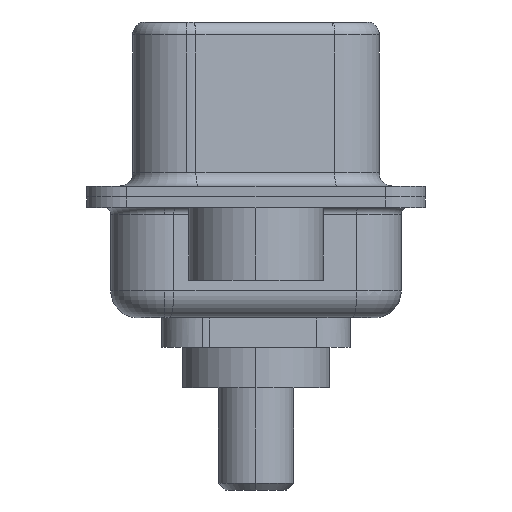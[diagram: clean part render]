
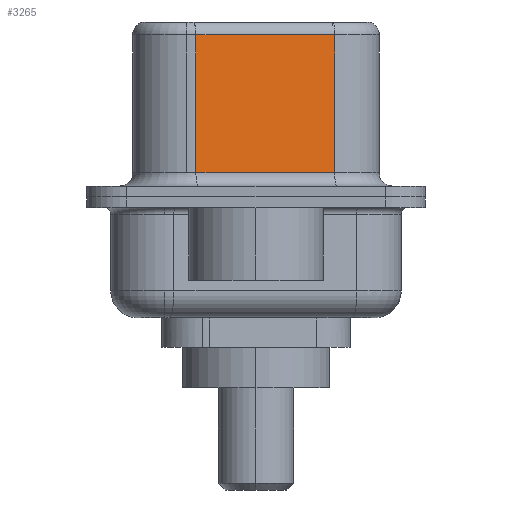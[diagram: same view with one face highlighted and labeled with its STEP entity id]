
A CAD part, left-side view. The second image highlights one B-rep face of the part: STEP entity #3265.
In plain terms, the highlighted planar face has unit normal (-0.985, -0.174, 0).
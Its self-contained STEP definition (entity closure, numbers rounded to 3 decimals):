
#342 = LINE ( 'NONE', #15076, #3213 ) ;
#769 = ORIENTED_EDGE ( 'NONE', *, *, #2416, .T. ) ;
#1430 = VECTOR ( 'NONE', #7669, 1000. ) ;
#1435 = EDGE_CURVE ( 'NONE', #5504, #11546, #342, .T. ) ;
#1739 = ORIENTED_EDGE ( 'NONE', *, *, #15233, .F. ) ;
#2416 = EDGE_CURVE ( 'NONE', #11546, #12562, #7179, .T. ) ;
#3213 = VECTOR ( 'NONE', #15706, 1000. ) ;
#3265 = ADVANCED_FACE ( 'NONE', ( #5222 ), #5969, .F. ) ;
#4072 = CARTESIAN_POINT ( 'NONE',  ( 4.58, -2.927, 6.52 ) ) ;
#5222 = FACE_OUTER_BOUND ( 'NONE', #7385, .T. ) ;
#5429 = DIRECTION ( 'NONE',  ( 0.174, -0.985, 0. ) ) ;
#5481 = LINE ( 'NONE', #11770, #8180 ) ;
#5504 = VERTEX_POINT ( 'NONE', #7075 ) ;
#5969 = PLANE ( 'NONE',  #13136 ) ;
#5988 = CARTESIAN_POINT ( 'NONE',  ( 3.67, 2.233, 6.02 ) ) ;
#6196 = CARTESIAN_POINT ( 'NONE',  ( 4.58, -2.927, 0.9 ) ) ;
#7075 = CARTESIAN_POINT ( 'NONE',  ( 4.58, -2.927, 6.02 ) ) ;
#7142 = CARTESIAN_POINT ( 'NONE',  ( 4.58, -2.927, 6.52 ) ) ;
#7179 = LINE ( 'NONE', #14147, #14959 ) ;
#7385 = EDGE_LOOP ( 'NONE', ( #1739, #12384, #769, #7457 ) ) ;
#7457 = ORIENTED_EDGE ( 'NONE', *, *, #14735, .T. ) ;
#7669 = DIRECTION ( 'NONE',  ( 0., 0., -1. ) ) ;
#8180 = VECTOR ( 'NONE', #5429, 1000. ) ;
#9249 = VERTEX_POINT ( 'NONE', #6196 ) ;
#9379 = LINE ( 'NONE', #4072, #1430 ) ;
#10450 = DIRECTION ( 'NONE',  ( 0., 0., -1. ) ) ;
#10930 = DIRECTION ( 'NONE',  ( 0.985, 0.174, 0. ) ) ;
#11546 = VERTEX_POINT ( 'NONE', #5988 ) ;
#11770 = CARTESIAN_POINT ( 'NONE',  ( 4.58, -2.927, 0.9 ) ) ;
#12384 = ORIENTED_EDGE ( 'NONE', *, *, #1435, .T. ) ;
#12562 = VERTEX_POINT ( 'NONE', #15073 ) ;
#13136 = AXIS2_PLACEMENT_3D ( 'NONE', #7142, #10930, #15829 ) ;
#14147 = CARTESIAN_POINT ( 'NONE',  ( 3.67, 2.233, 6.52 ) ) ;
#14735 = EDGE_CURVE ( 'NONE', #12562, #9249, #5481, .T. ) ;
#14959 = VECTOR ( 'NONE', #10450, 1000. ) ;
#15073 = CARTESIAN_POINT ( 'NONE',  ( 3.67, 2.233, 0.9 ) ) ;
#15076 = CARTESIAN_POINT ( 'NONE',  ( 4.58, -2.927, 6.02 ) ) ;
#15233 = EDGE_CURVE ( 'NONE', #5504, #9249, #9379, .T. ) ;
#15706 = DIRECTION ( 'NONE',  ( -0.174, 0.985, 0. ) ) ;
#15829 = DIRECTION ( 'NONE',  ( -0.174, 0.985, 0. ) ) ;
